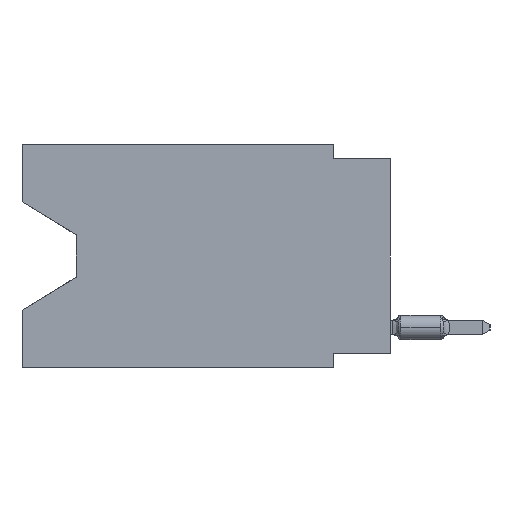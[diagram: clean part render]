
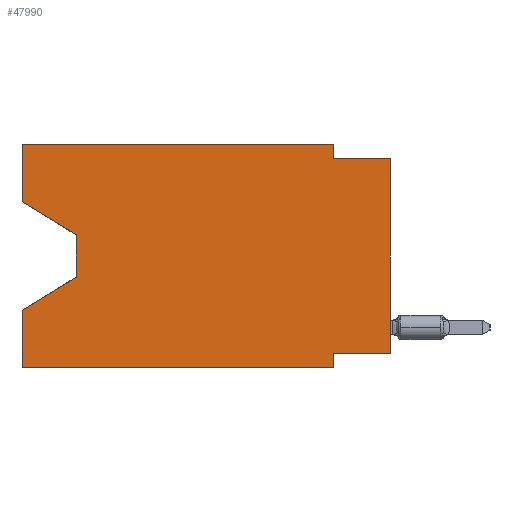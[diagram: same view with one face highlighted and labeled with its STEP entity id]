
A CAD part, left-side view. The second image highlights one B-rep face of the part: STEP entity #47990.
In plain terms, the highlighted planar face has unit normal (-1, 0, 0).
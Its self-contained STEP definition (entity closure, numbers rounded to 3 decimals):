
#1043 = VECTOR ( 'NONE', #63328, 1000. ) ;
#1196 = ORIENTED_EDGE ( 'NONE', *, *, #9870, .F. ) ;
#2636 = CARTESIAN_POINT ( 'NONE',  ( 0., 13.97, -4.013 ) ) ;
#2697 = CARTESIAN_POINT ( 'NONE',  ( 0., 2.54, 0. ) ) ;
#2984 = LINE ( 'NONE', #2636, #26832 ) ;
#3405 = CARTESIAN_POINT ( 'NONE',  ( 0., 13.97, -5.893 ) ) ;
#5241 = LINE ( 'NONE', #17397, #71708 ) ;
#5872 = CARTESIAN_POINT ( 'NONE',  ( 0., 16.383, 0. ) ) ;
#6094 = LINE ( 'NONE', #23436, #33490 ) ;
#7941 = ORIENTED_EDGE ( 'NONE', *, *, #23028, .F. ) ;
#8898 = DIRECTION ( 'NONE',  ( 1., 0., 0. ) ) ;
#9247 = CARTESIAN_POINT ( 'NONE',  ( 0., 0., -0.635 ) ) ;
#9799 = LINE ( 'NONE', #26754, #18880 ) ;
#9870 = EDGE_CURVE ( 'NONE', #19073, #60927, #6094, .T. ) ;
#11423 = CARTESIAN_POINT ( 'NONE',  ( 0., 16.383, -2.546 ) ) ;
#12275 = CARTESIAN_POINT ( 'NONE',  ( 0., 16.383, 0. ) ) ;
#12520 = LINE ( 'NONE', #5872, #68285 ) ;
#13091 = LINE ( 'NONE', #56697, #24365 ) ;
#13165 = CARTESIAN_POINT ( 'NONE',  ( 0., 2.54, -0.635 ) ) ;
#13611 = CARTESIAN_POINT ( 'NONE',  ( 0., 16.383, -9.906 ) ) ;
#13878 = VECTOR ( 'NONE', #45850, 1000. ) ;
#14847 = EDGE_LOOP ( 'NONE', ( #65335, #15475, #55760, #7941, #27301, #1196, #48055, #33593, #19815, #34418, #30364, #64799 ) ) ;
#14952 = CARTESIAN_POINT ( 'NONE',  ( 0., 0., -0.635 ) ) ;
#15475 = ORIENTED_EDGE ( 'NONE', *, *, #38225, .T. ) ;
#16972 = LINE ( 'NONE', #11423, #19225 ) ;
#17397 = CARTESIAN_POINT ( 'NONE',  ( 0., 16.383, -9.906 ) ) ;
#17422 = FACE_OUTER_BOUND ( 'NONE', #14847, .T. ) ;
#18353 = AXIS2_PLACEMENT_3D ( 'NONE', #45496, #8898, #64329 ) ;
#18880 = VECTOR ( 'NONE', #60400, 1000. ) ;
#19073 = VERTEX_POINT ( 'NONE', #59780 ) ;
#19225 = VECTOR ( 'NONE', #72746, 1000. ) ;
#19338 = CARTESIAN_POINT ( 'NONE',  ( 0., 16.383, -7.36 ) ) ;
#19815 = ORIENTED_EDGE ( 'NONE', *, *, #23990, .F. ) ;
#21232 = VERTEX_POINT ( 'NONE', #3405 ) ;
#21977 = DIRECTION ( 'NONE',  ( 0., 0., -1. ) ) ;
#22968 = PLANE ( 'NONE',  #18353 ) ;
#23028 = EDGE_CURVE ( 'NONE', #46791, #36476, #12520, .T. ) ;
#23436 = CARTESIAN_POINT ( 'NONE',  ( 0., 2.54, -9.906 ) ) ;
#23666 = EDGE_CURVE ( 'NONE', #72944, #19073, #9799, .T. ) ;
#23990 = EDGE_CURVE ( 'NONE', #37243, #53015, #25863, .T. ) ;
#24365 = VECTOR ( 'NONE', #68500, 1000. ) ;
#25663 = LINE ( 'NONE', #41928, #54904 ) ;
#25863 = LINE ( 'NONE', #9247, #56587 ) ;
#26754 = CARTESIAN_POINT ( 'NONE',  ( 0., 0., -9.271 ) ) ;
#26832 = VECTOR ( 'NONE', #54318, 1000. ) ;
#26881 = VECTOR ( 'NONE', #39415, 1000. ) ;
#27301 = ORIENTED_EDGE ( 'NONE', *, *, #51983, .T. ) ;
#27885 = EDGE_CURVE ( 'NONE', #66144, #65792, #16972, .T. ) ;
#28850 = CARTESIAN_POINT ( 'NONE',  ( 0., 2.54, -9.906 ) ) ;
#28855 = DIRECTION ( 'NONE',  ( 0., -1., 0. ) ) ;
#30364 = ORIENTED_EDGE ( 'NONE', *, *, #63883, .F. ) ;
#32337 = CARTESIAN_POINT ( 'NONE',  ( 0., 16.383, -2.546 ) ) ;
#33490 = VECTOR ( 'NONE', #21977, 1000. ) ;
#33517 = CARTESIAN_POINT ( 'NONE',  ( 0., 13.97, -5.893 ) ) ;
#33593 = ORIENTED_EDGE ( 'NONE', *, *, #48739, .T. ) ;
#34418 = ORIENTED_EDGE ( 'NONE', *, *, #61284, .F. ) ;
#36476 = VERTEX_POINT ( 'NONE', #19338 ) ;
#37243 = VERTEX_POINT ( 'NONE', #13165 ) ;
#37967 = VERTEX_POINT ( 'NONE', #66588 ) ;
#38225 = EDGE_CURVE ( 'NONE', #65792, #21232, #2984, .T. ) ;
#39415 = DIRECTION ( 'NONE',  ( 0., 0.855, -0.519 ) ) ;
#39850 = EDGE_CURVE ( 'NONE', #66144, #37967, #66787, .T. ) ;
#41928 = CARTESIAN_POINT ( 'NONE',  ( 0., 2.54, 0. ) ) ;
#43130 = CARTESIAN_POINT ( 'NONE',  ( 0., 13.97, -4.013 ) ) ;
#44782 = VERTEX_POINT ( 'NONE', #2697 ) ;
#45496 = CARTESIAN_POINT ( 'NONE',  ( 0., 16.383, 0. ) ) ;
#45850 = DIRECTION ( 'NONE',  ( 0., -1., 0. ) ) ;
#46791 = VERTEX_POINT ( 'NONE', #13611 ) ;
#46836 = DIRECTION ( 'NONE',  ( 0., 0., 1. ) ) ;
#47990 = ADVANCED_FACE ( 'NONE', ( #17422 ), #22968, .F. ) ;
#48055 = ORIENTED_EDGE ( 'NONE', *, *, #23666, .F. ) ;
#48189 = CARTESIAN_POINT ( 'NONE',  ( 0., 0., -9.271 ) ) ;
#48739 = EDGE_CURVE ( 'NONE', #72944, #53015, #13091, .T. ) ;
#48764 = DIRECTION ( 'NONE',  ( 0., -1., 0. ) ) ;
#50675 = LINE ( 'NONE', #12275, #13878 ) ;
#51983 = EDGE_CURVE ( 'NONE', #46791, #60927, #5241, .T. ) ;
#52265 = CARTESIAN_POINT ( 'NONE',  ( 0., 16.383, 0. ) ) ;
#53015 = VERTEX_POINT ( 'NONE', #14952 ) ;
#54318 = DIRECTION ( 'NONE',  ( 0., 0., -1. ) ) ;
#54904 = VECTOR ( 'NONE', #57847, 1000. ) ;
#55760 = ORIENTED_EDGE ( 'NONE', *, *, #64673, .T. ) ;
#56587 = VECTOR ( 'NONE', #48764, 1000. ) ;
#56697 = CARTESIAN_POINT ( 'NONE',  ( 0., 0., 0. ) ) ;
#57847 = DIRECTION ( 'NONE',  ( 0., 0., -1. ) ) ;
#59780 = CARTESIAN_POINT ( 'NONE',  ( 0., 2.54, -9.271 ) ) ;
#60400 = DIRECTION ( 'NONE',  ( 0., 1., 0. ) ) ;
#60927 = VERTEX_POINT ( 'NONE', #28850 ) ;
#61284 = EDGE_CURVE ( 'NONE', #44782, #37243, #25663, .T. ) ;
#63328 = DIRECTION ( 'NONE',  ( 0., 0., 1. ) ) ;
#63883 = EDGE_CURVE ( 'NONE', #37967, #44782, #50675, .T. ) ;
#64329 = DIRECTION ( 'NONE',  ( 0., 0., -1. ) ) ;
#64673 = EDGE_CURVE ( 'NONE', #21232, #36476, #73040, .T. ) ;
#64799 = ORIENTED_EDGE ( 'NONE', *, *, #39850, .F. ) ;
#65335 = ORIENTED_EDGE ( 'NONE', *, *, #27885, .T. ) ;
#65792 = VERTEX_POINT ( 'NONE', #43130 ) ;
#66144 = VERTEX_POINT ( 'NONE', #32337 ) ;
#66588 = CARTESIAN_POINT ( 'NONE',  ( 0., 16.383, 0. ) ) ;
#66787 = LINE ( 'NONE', #52265, #1043 ) ;
#68285 = VECTOR ( 'NONE', #46836, 1000. ) ;
#68500 = DIRECTION ( 'NONE',  ( 0., 0., 1. ) ) ;
#71708 = VECTOR ( 'NONE', #28855, 1000. ) ;
#72746 = DIRECTION ( 'NONE',  ( 0., -0.855, -0.519 ) ) ;
#72944 = VERTEX_POINT ( 'NONE', #48189 ) ;
#73040 = LINE ( 'NONE', #33517, #26881 ) ;
